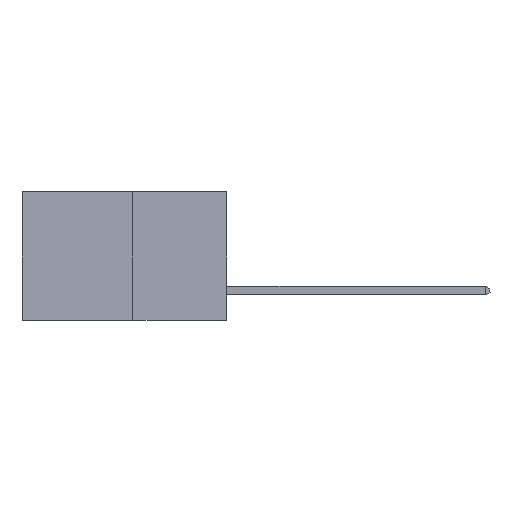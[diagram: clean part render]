
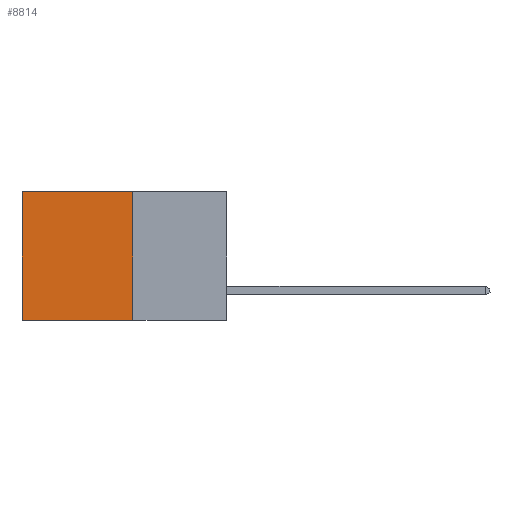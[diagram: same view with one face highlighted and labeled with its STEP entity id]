
A CAD part, left-side view. The second image highlights one B-rep face of the part: STEP entity #8814.
In plain terms, the highlighted planar face has unit normal (-1, 0, 0).
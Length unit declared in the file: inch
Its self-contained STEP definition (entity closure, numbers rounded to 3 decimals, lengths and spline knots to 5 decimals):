
#654 = PLANE ( 'NONE',  #8825 ) ;
#851 = DIRECTION ( 'NONE',  ( 0., 0., -1. ) ) ;
#1901 = DIRECTION ( 'NONE',  ( 0., 1., 0. ) ) ;
#1917 = CARTESIAN_POINT ( 'NONE',  ( 0.277, 0.59, -0.37 ) ) ;
#2063 = CARTESIAN_POINT ( 'NONE',  ( 0.277, 0.59, -0.37 ) ) ;
#2343 = VECTOR ( 'NONE', #1901, 39.37008 ) ;
#2914 = ORIENTED_EDGE ( 'NONE', *, *, #16305, .T. ) ;
#3341 = CARTESIAN_POINT ( 'NONE',  ( 0.277, 0.27, -0.37 ) ) ;
#3409 = DIRECTION ( 'NONE',  ( 0., 0., -1. ) ) ;
#3605 = LINE ( 'NONE', #7498, #13856 ) ;
#4687 = DIRECTION ( 'NONE',  ( 0., 0., -1. ) ) ;
#4744 = VECTOR ( 'NONE', #13589, 39.37008 ) ;
#4817 = VERTEX_POINT ( 'NONE', #7641 ) ;
#5583 = CARTESIAN_POINT ( 'NONE',  ( 0.277, 0.27, 0. ) ) ;
#5757 = EDGE_LOOP ( 'NONE', ( #7181, #16062, #7980, #2914 ) ) ;
#6080 = EDGE_CURVE ( 'NONE', #4817, #10688, #12538, .T. ) ;
#6612 = FACE_OUTER_BOUND ( 'NONE', #5757, .T. ) ;
#7181 = ORIENTED_EDGE ( 'NONE', *, *, #6080, .T. ) ;
#7498 = CARTESIAN_POINT ( 'NONE',  ( 0.277, 0.27, -0.37 ) ) ;
#7527 = CARTESIAN_POINT ( 'NONE',  ( 0.277, 0.27, 0. ) ) ;
#7558 = VERTEX_POINT ( 'NONE', #10518 ) ;
#7641 = CARTESIAN_POINT ( 'NONE',  ( 0.277, 0.59, 0. ) ) ;
#7980 = ORIENTED_EDGE ( 'NONE', *, *, #14031, .F. ) ;
#8814 = ADVANCED_FACE ( 'NONE', ( #6612 ), #654, .F. ) ;
#8825 = AXIS2_PLACEMENT_3D ( 'NONE', #3341, #12666, #4687 ) ;
#9013 = LINE ( 'NONE', #9856, #2343 ) ;
#9856 = CARTESIAN_POINT ( 'NONE',  ( 0.277, 0.27, -0.37 ) ) ;
#10518 = CARTESIAN_POINT ( 'NONE',  ( 0.277, 0.27, -0.37 ) ) ;
#10688 = VERTEX_POINT ( 'NONE', #1917 ) ;
#11411 = LINE ( 'NONE', #5583, #4744 ) ;
#12109 = VECTOR ( 'NONE', #3409, 39.37008 ) ;
#12538 = LINE ( 'NONE', #2063, #12109 ) ;
#12666 = DIRECTION ( 'NONE',  ( 1., 0., 0. ) ) ;
#13589 = DIRECTION ( 'NONE',  ( 0., 1., 0. ) ) ;
#13856 = VECTOR ( 'NONE', #851, 39.37008 ) ;
#14031 = EDGE_CURVE ( 'NONE', #17221, #7558, #3605, .T. ) ;
#14496 = EDGE_CURVE ( 'NONE', #7558, #10688, #9013, .T. ) ;
#16062 = ORIENTED_EDGE ( 'NONE', *, *, #14496, .F. ) ;
#16305 = EDGE_CURVE ( 'NONE', #17221, #4817, #11411, .T. ) ;
#17221 = VERTEX_POINT ( 'NONE', #7527 ) ;
